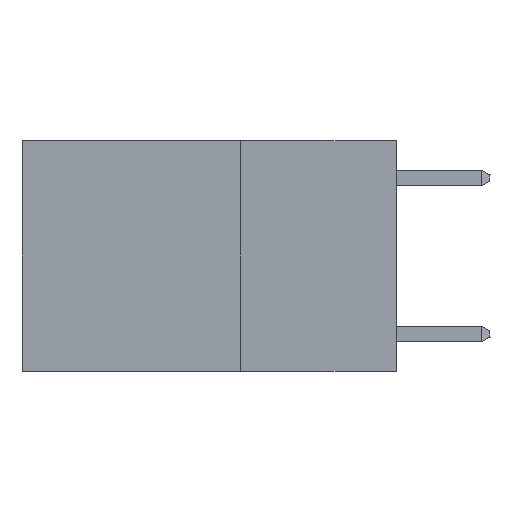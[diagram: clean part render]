
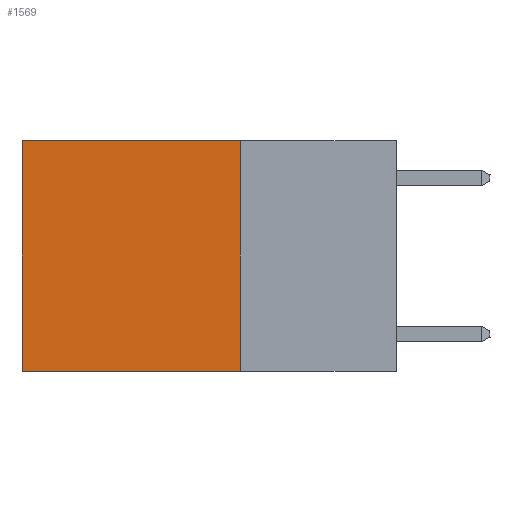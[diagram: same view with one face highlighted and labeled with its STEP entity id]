
A CAD part, left-side view. The second image highlights one B-rep face of the part: STEP entity #1569.
In plain terms, the highlighted planar face has unit normal (-1, 0, 0).
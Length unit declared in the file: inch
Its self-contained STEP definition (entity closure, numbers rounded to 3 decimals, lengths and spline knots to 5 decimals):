
#379 = FACE_OUTER_BOUND ( 'NONE', #15788, .T. ) ;
#838 = LINE ( 'NONE', #1419, #22701 ) ;
#957 = LINE ( 'NONE', #18266, #15250 ) ;
#1419 = CARTESIAN_POINT ( 'NONE',  ( 0.2625, 0.25, -0.37 ) ) ;
#1519 = AXIS2_PLACEMENT_3D ( 'NONE', #9025, #16072, #2130 ) ;
#1569 = ADVANCED_FACE ( 'NONE', ( #379 ), #7391, .F. ) ;
#1773 = VECTOR ( 'NONE', #2400, 39.37008 ) ;
#2130 = DIRECTION ( 'NONE',  ( 0., 0., -1. ) ) ;
#2400 = DIRECTION ( 'NONE',  ( 0., 1., 0. ) ) ;
#2918 = DIRECTION ( 'NONE',  ( 0., 1., 0. ) ) ;
#3900 = ORIENTED_EDGE ( 'NONE', *, *, #7242, .F. ) ;
#3962 = CARTESIAN_POINT ( 'NONE',  ( 0.2625, 0.6, 0. ) ) ;
#4194 = VERTEX_POINT ( 'NONE', #22705 ) ;
#6055 = CARTESIAN_POINT ( 'NONE',  ( 0.2625, 0.25, 0. ) ) ;
#7242 = EDGE_CURVE ( 'NONE', #4194, #17397, #838, .T. ) ;
#7391 = PLANE ( 'NONE',  #1519 ) ;
#8178 = EDGE_CURVE ( 'NONE', #20556, #8415, #15164, .T. ) ;
#8262 = CARTESIAN_POINT ( 'NONE',  ( 0.2625, 0.6, -0.37 ) ) ;
#8415 = VERTEX_POINT ( 'NONE', #3962 ) ;
#9008 = ORIENTED_EDGE ( 'NONE', *, *, #15011, .F. ) ;
#9025 = CARTESIAN_POINT ( 'NONE',  ( 0.2625, 0.25, 0. ) ) ;
#11936 = LINE ( 'NONE', #19006, #12090 ) ;
#12090 = VECTOR ( 'NONE', #15531, 39.37008 ) ;
#12338 = CARTESIAN_POINT ( 'NONE',  ( 0.2625, 0.25, 0. ) ) ;
#15011 = EDGE_CURVE ( 'NONE', #20556, #4194, #957, .T. ) ;
#15164 = LINE ( 'NONE', #6055, #1773 ) ;
#15250 = VECTOR ( 'NONE', #22179, 39.37008 ) ;
#15531 = DIRECTION ( 'NONE',  ( 0., 0., -1. ) ) ;
#15788 = EDGE_LOOP ( 'NONE', ( #20210, #3900, #9008, #21045 ) ) ;
#16072 = DIRECTION ( 'NONE',  ( 1., 0., 0. ) ) ;
#17397 = VERTEX_POINT ( 'NONE', #8262 ) ;
#18266 = CARTESIAN_POINT ( 'NONE',  ( 0.2625, 0.25, 0. ) ) ;
#19006 = CARTESIAN_POINT ( 'NONE',  ( 0.2625, 0.6, 0. ) ) ;
#20210 = ORIENTED_EDGE ( 'NONE', *, *, #20927, .T. ) ;
#20556 = VERTEX_POINT ( 'NONE', #12338 ) ;
#20927 = EDGE_CURVE ( 'NONE', #8415, #17397, #11936, .T. ) ;
#21045 = ORIENTED_EDGE ( 'NONE', *, *, #8178, .T. ) ;
#22179 = DIRECTION ( 'NONE',  ( 0., 0., -1. ) ) ;
#22701 = VECTOR ( 'NONE', #2918, 39.37008 ) ;
#22705 = CARTESIAN_POINT ( 'NONE',  ( 0.2625, 0.25, -0.37 ) ) ;
